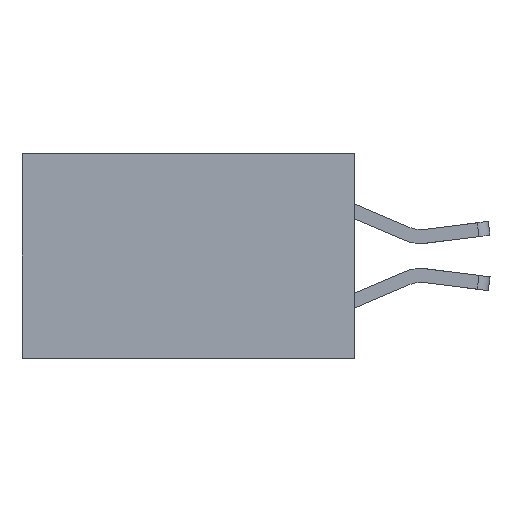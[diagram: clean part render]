
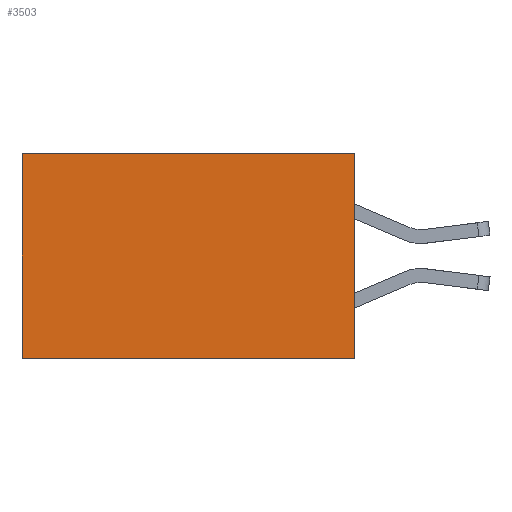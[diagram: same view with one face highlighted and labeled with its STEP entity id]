
A CAD part, left-side view. The second image highlights one B-rep face of the part: STEP entity #3503.
In plain terms, the highlighted planar face has unit normal (-1, 0, 0).
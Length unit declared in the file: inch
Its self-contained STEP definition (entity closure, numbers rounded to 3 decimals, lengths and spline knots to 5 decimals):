
#96 = DIRECTION ( 'NONE',  ( 1., 0., 0. ) ) ;
#356 = LINE ( 'NONE', #12201, #6888 ) ;
#561 = VERTEX_POINT ( 'NONE', #11422 ) ;
#1342 = DIRECTION ( 'NONE',  ( 0., 1., 0. ) ) ;
#1700 = EDGE_CURVE ( 'NONE', #12136, #561, #356, .T. ) ;
#2216 = CARTESIAN_POINT ( 'NONE',  ( 0.298, 0., -0.37 ) ) ;
#2857 = CARTESIAN_POINT ( 'NONE',  ( 0.298, 0., 0. ) ) ;
#2905 = FACE_OUTER_BOUND ( 'NONE', #7895, .T. ) ;
#2921 = DIRECTION ( 'NONE',  ( 0., 0., -1. ) ) ;
#3285 = CARTESIAN_POINT ( 'NONE',  ( 0.298, 0.6, 0. ) ) ;
#3503 = ADVANCED_FACE ( 'NONE', ( #2905 ), #12475, .F. ) ;
#3747 = CARTESIAN_POINT ( 'NONE',  ( 0.298, 0., 0. ) ) ;
#4147 = CARTESIAN_POINT ( 'NONE',  ( 0.298, 0., -0.37 ) ) ;
#4343 = VECTOR ( 'NONE', #2921, 39.37008 ) ;
#5189 = DIRECTION ( 'NONE',  ( 0., 1., 0. ) ) ;
#5738 = ORIENTED_EDGE ( 'NONE', *, *, #7364, .F. ) ;
#6492 = VECTOR ( 'NONE', #5189, 39.37008 ) ;
#6888 = VECTOR ( 'NONE', #1342, 39.37008 ) ;
#6986 = EDGE_CURVE ( 'NONE', #561, #8894, #10467, .T. ) ;
#7364 = EDGE_CURVE ( 'NONE', #12136, #11248, #11176, .T. ) ;
#7714 = VECTOR ( 'NONE', #10015, 39.37008 ) ;
#7716 = EDGE_CURVE ( 'NONE', #11248, #8894, #9674, .T. ) ;
#7895 = EDGE_LOOP ( 'NONE', ( #12126, #12058, #5738, #12609 ) ) ;
#8894 = VERTEX_POINT ( 'NONE', #11142 ) ;
#9126 = AXIS2_PLACEMENT_3D ( 'NONE', #2857, #96, #10730 ) ;
#9674 = LINE ( 'NONE', #4147, #6492 ) ;
#10015 = DIRECTION ( 'NONE',  ( 0., 0., -1. ) ) ;
#10467 = LINE ( 'NONE', #3285, #7714 ) ;
#10730 = DIRECTION ( 'NONE',  ( 0., 0., -1. ) ) ;
#11142 = CARTESIAN_POINT ( 'NONE',  ( 0.298, 0.6, -0.37 ) ) ;
#11176 = LINE ( 'NONE', #12580, #4343 ) ;
#11248 = VERTEX_POINT ( 'NONE', #2216 ) ;
#11422 = CARTESIAN_POINT ( 'NONE',  ( 0.298, 0.6, 0. ) ) ;
#12058 = ORIENTED_EDGE ( 'NONE', *, *, #7716, .F. ) ;
#12126 = ORIENTED_EDGE ( 'NONE', *, *, #6986, .T. ) ;
#12136 = VERTEX_POINT ( 'NONE', #3747 ) ;
#12201 = CARTESIAN_POINT ( 'NONE',  ( 0.298, 0., 0. ) ) ;
#12475 = PLANE ( 'NONE',  #9126 ) ;
#12580 = CARTESIAN_POINT ( 'NONE',  ( 0.298, 0., 0. ) ) ;
#12609 = ORIENTED_EDGE ( 'NONE', *, *, #1700, .T. ) ;
